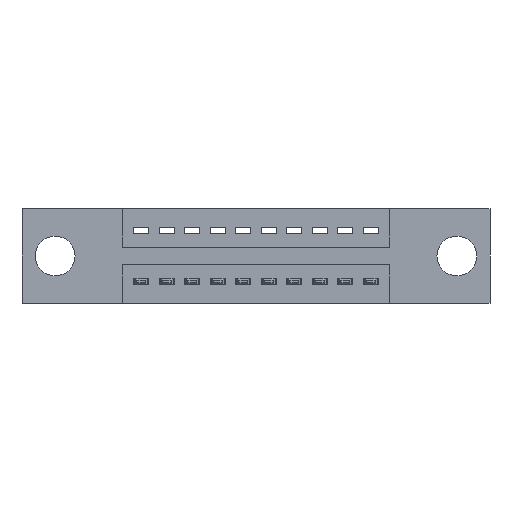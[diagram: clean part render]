
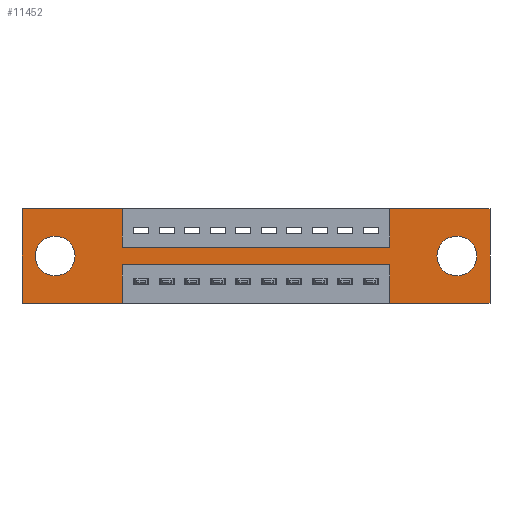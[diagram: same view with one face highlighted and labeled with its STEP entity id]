
A CAD part, front view. The second image highlights one B-rep face of the part: STEP entity #11452.
In plain terms, the highlighted planar face has unit normal (0, -1, 0).
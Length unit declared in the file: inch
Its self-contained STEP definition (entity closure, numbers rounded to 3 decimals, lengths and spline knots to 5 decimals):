
#127 = AXIS2_PLACEMENT_3D ( 'NONE', #5581, #3660, #7404 ) ;
#136 = EDGE_CURVE ( 'NONE', #5483, #7820, #4250, .T. ) ;
#151 = VECTOR ( 'NONE', #576, 39.37008 ) ;
#372 = ORIENTED_EDGE ( 'NONE', *, *, #1850, .F. ) ;
#491 = VERTEX_POINT ( 'NONE', #5455 ) ;
#576 = DIRECTION ( 'NONE',  ( 0., 0., 1. ) ) ;
#710 = CARTESIAN_POINT ( 'NONE',  ( 1.4425, 0., -0.22 ) ) ;
#801 = DIRECTION ( 'NONE',  ( 1., 0., 0. ) ) ;
#864 = CARTESIAN_POINT ( 'NONE',  ( 0., 0., 0. ) ) ;
#1239 = AXIS2_PLACEMENT_3D ( 'NONE', #6769, #10498, #6710 ) ;
#1261 = ORIENTED_EDGE ( 'NONE', *, *, #5811, .F. ) ;
#1372 = LINE ( 'NONE', #7122, #151 ) ;
#1439 = ORIENTED_EDGE ( 'NONE', *, *, #6889, .F. ) ;
#1556 = EDGE_CURVE ( 'NONE', #7876, #491, #5820, .T. ) ;
#1576 = VERTEX_POINT ( 'NONE', #6578 ) ;
#1850 = EDGE_CURVE ( 'NONE', #11626, #10175, #1372, .T. ) ;
#2020 = DIRECTION ( 'NONE',  ( 1., 0., 0. ) ) ;
#2027 = VECTOR ( 'NONE', #4925, 39.37008 ) ;
#2401 = FACE_BOUND ( 'NONE', #11651, .T. ) ;
#2581 = VERTEX_POINT ( 'NONE', #4256 ) ;
#2693 = DIRECTION ( 'NONE',  ( 0., 0., 1. ) ) ;
#2793 = VERTEX_POINT ( 'NONE', #10478 ) ;
#2976 = FACE_OUTER_BOUND ( 'NONE', #11412, .T. ) ;
#3287 = LINE ( 'NONE', #7025, #10074 ) ;
#3335 = CARTESIAN_POINT ( 'NONE',  ( 1.835, 0., 0. ) ) ;
#3434 = CARTESIAN_POINT ( 'NONE',  ( 0.13, 0., -0.185 ) ) ;
#3453 = EDGE_CURVE ( 'NONE', #7820, #2793, #7170, .T. ) ;
#3499 = DIRECTION ( 'NONE',  ( -1., 0., 0. ) ) ;
#3508 = ORIENTED_EDGE ( 'NONE', *, *, #3453, .F. ) ;
#3613 = CARTESIAN_POINT ( 'NONE',  ( 0., 0., -0.37 ) ) ;
#3617 = EDGE_CURVE ( 'NONE', #2581, #7302, #8134, .T. ) ;
#3627 = VECTOR ( 'NONE', #9942, 39.37008 ) ;
#3660 = DIRECTION ( 'NONE',  ( 0., 1., 0. ) ) ;
#3705 = CARTESIAN_POINT ( 'NONE',  ( 1.4425, 0., -0.37 ) ) ;
#3720 = CARTESIAN_POINT ( 'NONE',  ( 1.4425, 0., -0.15 ) ) ;
#3747 = VERTEX_POINT ( 'NONE', #7086 ) ;
#3760 = ORIENTED_EDGE ( 'NONE', *, *, #8175, .T. ) ;
#3773 = EDGE_CURVE ( 'NONE', #10442, #3747, #3287, .T. ) ;
#4119 = VERTEX_POINT ( 'NONE', #3335 ) ;
#4125 = CARTESIAN_POINT ( 'NONE',  ( 0.3925, 0., 0. ) ) ;
#4234 = LINE ( 'NONE', #7177, #8566 ) ;
#4250 = LINE ( 'NONE', #11724, #5337 ) ;
#4256 = CARTESIAN_POINT ( 'NONE',  ( 0.13, 0., -0.263 ) ) ;
#4278 = ORIENTED_EDGE ( 'NONE', *, *, #7637, .F. ) ;
#4281 = EDGE_CURVE ( 'NONE', #1576, #4119, #9996, .T. ) ;
#4334 = ORIENTED_EDGE ( 'NONE', *, *, #5898, .T. ) ;
#4345 = EDGE_CURVE ( 'NONE', #4119, #10442, #9564, .T. ) ;
#4550 = CARTESIAN_POINT ( 'NONE',  ( 0.13, 0., -0.107 ) ) ;
#4805 = ORIENTED_EDGE ( 'NONE', *, *, #3617, .T. ) ;
#4925 = DIRECTION ( 'NONE',  ( 0., 0., -1. ) ) ;
#5028 = VECTOR ( 'NONE', #8641, 39.37008 ) ;
#5131 = ORIENTED_EDGE ( 'NONE', *, *, #136, .F. ) ;
#5230 = CARTESIAN_POINT ( 'NONE',  ( 0., 0., 0. ) ) ;
#5263 = VECTOR ( 'NONE', #7584, 39.37008 ) ;
#5337 = VECTOR ( 'NONE', #3499, 39.37008 ) ;
#5339 = ORIENTED_EDGE ( 'NONE', *, *, #3773, .F. ) ;
#5455 = CARTESIAN_POINT ( 'NONE',  ( 1.705, 0., -0.263 ) ) ;
#5483 = VERTEX_POINT ( 'NONE', #710 ) ;
#5581 = CARTESIAN_POINT ( 'NONE',  ( 0.13, 0., -0.185 ) ) ;
#5786 = CARTESIAN_POINT ( 'NONE',  ( 0.3925, 0., 0. ) ) ;
#5811 = EDGE_CURVE ( 'NONE', #10742, #10952, #7347, .T. ) ;
#5820 = CIRCLE ( 'NONE', #10681, 0.078 ) ;
#5842 = CIRCLE ( 'NONE', #7396, 0.078 ) ;
#5847 = LINE ( 'NONE', #5786, #2027 ) ;
#5898 = EDGE_CURVE ( 'NONE', #7302, #2581, #9145, .T. ) ;
#6216 = FACE_BOUND ( 'NONE', #9399, .T. ) ;
#6221 = CARTESIAN_POINT ( 'NONE',  ( 0., 0., 0. ) ) ;
#6460 = EDGE_CURVE ( 'NONE', #2793, #11626, #6718, .T. ) ;
#6578 = CARTESIAN_POINT ( 'NONE',  ( 1.4425, 0., 0. ) ) ;
#6593 = LINE ( 'NONE', #3705, #9328 ) ;
#6710 = DIRECTION ( 'NONE',  ( 0., 0., -1. ) ) ;
#6718 = LINE ( 'NONE', #9537, #5263 ) ;
#6769 = CARTESIAN_POINT ( 'NONE',  ( 0., 0., -0.37 ) ) ;
#6889 = EDGE_CURVE ( 'NONE', #3747, #5483, #6593, .T. ) ;
#6923 = CARTESIAN_POINT ( 'NONE',  ( 0.3925, 0., -0.37 ) ) ;
#7025 = CARTESIAN_POINT ( 'NONE',  ( 0., 0., -0.37 ) ) ;
#7051 = VERTEX_POINT ( 'NONE', #4125 ) ;
#7083 = ORIENTED_EDGE ( 'NONE', *, *, #9211, .F. ) ;
#7086 = CARTESIAN_POINT ( 'NONE',  ( 1.4425, 0., -0.37 ) ) ;
#7122 = CARTESIAN_POINT ( 'NONE',  ( 0., 0., 0. ) ) ;
#7170 = LINE ( 'NONE', #6923, #11641 ) ;
#7177 = CARTESIAN_POINT ( 'NONE',  ( 1.4425, 0., 0. ) ) ;
#7203 = VECTOR ( 'NONE', #801, 39.37008 ) ;
#7302 = VERTEX_POINT ( 'NONE', #4550 ) ;
#7347 = LINE ( 'NONE', #8269, #7203 ) ;
#7371 = CARTESIAN_POINT ( 'NONE',  ( 1.705, 0., -0.185 ) ) ;
#7396 = AXIS2_PLACEMENT_3D ( 'NONE', #11042, #11849, #8183 ) ;
#7404 = DIRECTION ( 'NONE',  ( 0., 0., 1. ) ) ;
#7446 = DIRECTION ( 'NONE',  ( 0., 0., 1. ) ) ;
#7584 = DIRECTION ( 'NONE',  ( -1., 0., 0. ) ) ;
#7637 = EDGE_CURVE ( 'NONE', #10952, #1576, #4234, .T. ) ;
#7820 = VERTEX_POINT ( 'NONE', #10449 ) ;
#7876 = VERTEX_POINT ( 'NONE', #10445 ) ;
#8063 = ORIENTED_EDGE ( 'NONE', *, *, #6460, .F. ) ;
#8134 = CIRCLE ( 'NONE', #127, 0.078 ) ;
#8175 = EDGE_CURVE ( 'NONE', #491, #7876, #5842, .T. ) ;
#8183 = DIRECTION ( 'NONE',  ( 0., 0., -1. ) ) ;
#8269 = CARTESIAN_POINT ( 'NONE',  ( 0.3925, 0., -0.15 ) ) ;
#8330 = DIRECTION ( 'NONE',  ( 0., 1., 0. ) ) ;
#8411 = CARTESIAN_POINT ( 'NONE',  ( 1.835, 0., 0. ) ) ;
#8566 = VECTOR ( 'NONE', #10205, 39.37008 ) ;
#8641 = DIRECTION ( 'NONE',  ( 0., 0., -1. ) ) ;
#8893 = PLANE ( 'NONE',  #1239 ) ;
#9000 = CARTESIAN_POINT ( 'NONE',  ( 0.3925, 0., -0.15 ) ) ;
#9091 = DIRECTION ( 'NONE',  ( -1., 0., 0. ) ) ;
#9145 = CIRCLE ( 'NONE', #9541, 0.078 ) ;
#9175 = ORIENTED_EDGE ( 'NONE', *, *, #4281, .F. ) ;
#9211 = EDGE_CURVE ( 'NONE', #10175, #7051, #10406, .T. ) ;
#9306 = CARTESIAN_POINT ( 'NONE',  ( 1.835, 0., -0.37 ) ) ;
#9328 = VECTOR ( 'NONE', #7446, 39.37008 ) ;
#9390 = DIRECTION ( 'NONE',  ( 0., 1., 0. ) ) ;
#9399 = EDGE_LOOP ( 'NONE', ( #10278, #3760 ) ) ;
#9537 = CARTESIAN_POINT ( 'NONE',  ( 0., 0., -0.37 ) ) ;
#9541 = AXIS2_PLACEMENT_3D ( 'NONE', #3434, #8330, #2693 ) ;
#9564 = LINE ( 'NONE', #8411, #5028 ) ;
#9578 = ORIENTED_EDGE ( 'NONE', *, *, #4345, .F. ) ;
#9764 = ORIENTED_EDGE ( 'NONE', *, *, #10019, .F. ) ;
#9942 = DIRECTION ( 'NONE',  ( 1., 0., 0. ) ) ;
#9996 = LINE ( 'NONE', #6221, #3627 ) ;
#10019 = EDGE_CURVE ( 'NONE', #7051, #10742, #5847, .T. ) ;
#10074 = VECTOR ( 'NONE', #9091, 39.37008 ) ;
#10175 = VERTEX_POINT ( 'NONE', #5230 ) ;
#10205 = DIRECTION ( 'NONE',  ( 0., 0., 1. ) ) ;
#10278 = ORIENTED_EDGE ( 'NONE', *, *, #1556, .T. ) ;
#10406 = LINE ( 'NONE', #864, #11529 ) ;
#10442 = VERTEX_POINT ( 'NONE', #9306 ) ;
#10445 = CARTESIAN_POINT ( 'NONE',  ( 1.705, 0., -0.107 ) ) ;
#10449 = CARTESIAN_POINT ( 'NONE',  ( 0.3925, 0., -0.22 ) ) ;
#10478 = CARTESIAN_POINT ( 'NONE',  ( 0.3925, 0., -0.37 ) ) ;
#10498 = DIRECTION ( 'NONE',  ( 0., -1., 0. ) ) ;
#10681 = AXIS2_PLACEMENT_3D ( 'NONE', #7371, #9390, #11098 ) ;
#10742 = VERTEX_POINT ( 'NONE', #9000 ) ;
#10894 = DIRECTION ( 'NONE',  ( 0., 0., -1. ) ) ;
#10952 = VERTEX_POINT ( 'NONE', #3720 ) ;
#11042 = CARTESIAN_POINT ( 'NONE',  ( 1.705, 0., -0.185 ) ) ;
#11098 = DIRECTION ( 'NONE',  ( 0., 0., -1. ) ) ;
#11412 = EDGE_LOOP ( 'NONE', ( #3508, #5131, #1439, #5339, #9578, #9175, #4278, #1261, #9764, #7083, #372, #8063 ) ) ;
#11452 = ADVANCED_FACE ( 'NONE', ( #6216, #2401, #2976 ), #8893, .T. ) ;
#11529 = VECTOR ( 'NONE', #2020, 39.37008 ) ;
#11626 = VERTEX_POINT ( 'NONE', #3613 ) ;
#11641 = VECTOR ( 'NONE', #10894, 39.37008 ) ;
#11651 = EDGE_LOOP ( 'NONE', ( #4334, #4805 ) ) ;
#11724 = CARTESIAN_POINT ( 'NONE',  ( 0.3925, 0., -0.22 ) ) ;
#11849 = DIRECTION ( 'NONE',  ( 0., 1., 0. ) ) ;
